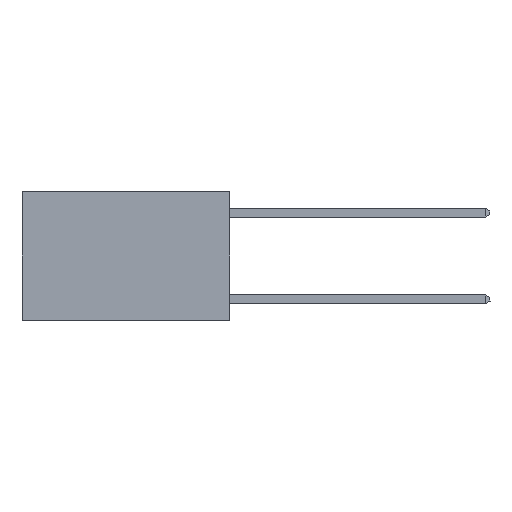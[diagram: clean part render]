
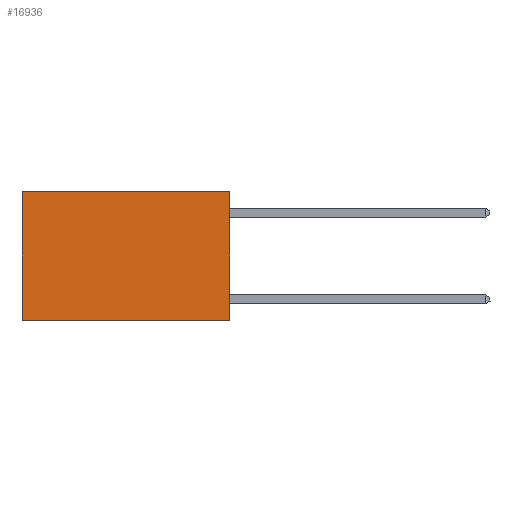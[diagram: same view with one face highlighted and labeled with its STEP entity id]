
A CAD part, left-side view. The second image highlights one B-rep face of the part: STEP entity #16936.
In plain terms, the highlighted planar face has unit normal (-1, 0, 0).
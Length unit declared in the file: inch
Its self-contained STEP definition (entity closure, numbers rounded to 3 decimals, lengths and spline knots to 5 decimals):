
#308 = ORIENTED_EDGE ( 'NONE', *, *, #13115, .T. ) ;
#621 = VERTEX_POINT ( 'NONE', #2435 ) ;
#2435 = CARTESIAN_POINT ( 'NONE',  ( 0.2625, 0., -0.37 ) ) ;
#2455 = VERTEX_POINT ( 'NONE', #16443 ) ;
#3854 = LINE ( 'NONE', #19638, #19950 ) ;
#4288 = DIRECTION ( 'NONE',  ( 0., 0., -1. ) ) ;
#4433 = LINE ( 'NONE', #13815, #7855 ) ;
#4659 = CARTESIAN_POINT ( 'NONE',  ( 0.2625, 0., 0. ) ) ;
#4822 = LINE ( 'NONE', #9016, #8762 ) ;
#6432 = PLANE ( 'NONE',  #19025 ) ;
#6442 = ORIENTED_EDGE ( 'NONE', *, *, #18600, .F. ) ;
#7121 = ORIENTED_EDGE ( 'NONE', *, *, #7258, .F. ) ;
#7258 = EDGE_CURVE ( 'NONE', #14819, #621, #4822, .T. ) ;
#7855 = VECTOR ( 'NONE', #15471, 39.37008 ) ;
#8762 = VECTOR ( 'NONE', #20571, 39.37008 ) ;
#9016 = CARTESIAN_POINT ( 'NONE',  ( 0.2625, 0., 0. ) ) ;
#9351 = CARTESIAN_POINT ( 'NONE',  ( 0.2625, 0.6, 0. ) ) ;
#9786 = DIRECTION ( 'NONE',  ( 1., 0., 0. ) ) ;
#10000 = CARTESIAN_POINT ( 'NONE',  ( 0.2625, 0.6, -0.37 ) ) ;
#11943 = LINE ( 'NONE', #9351, #15819 ) ;
#13093 = DIRECTION ( 'NONE',  ( 0., 1., 0. ) ) ;
#13115 = EDGE_CURVE ( 'NONE', #2455, #15050, #11943, .T. ) ;
#13815 = CARTESIAN_POINT ( 'NONE',  ( 0.2625, 0., 0. ) ) ;
#14245 = CARTESIAN_POINT ( 'NONE',  ( 0.2625, 0., 0. ) ) ;
#14819 = VERTEX_POINT ( 'NONE', #14245 ) ;
#15050 = VERTEX_POINT ( 'NONE', #10000 ) ;
#15471 = DIRECTION ( 'NONE',  ( 0., 1., 0. ) ) ;
#15819 = VECTOR ( 'NONE', #4288, 39.37008 ) ;
#16443 = CARTESIAN_POINT ( 'NONE',  ( 0.2625, 0.6, 0. ) ) ;
#16548 = EDGE_CURVE ( 'NONE', #14819, #2455, #4433, .T. ) ;
#16727 = EDGE_LOOP ( 'NONE', ( #308, #6442, #7121, #17987 ) ) ;
#16936 = ADVANCED_FACE ( 'NONE', ( #17171 ), #6432, .F. ) ;
#17171 = FACE_OUTER_BOUND ( 'NONE', #16727, .T. ) ;
#17987 = ORIENTED_EDGE ( 'NONE', *, *, #16548, .T. ) ;
#18600 = EDGE_CURVE ( 'NONE', #621, #15050, #3854, .T. ) ;
#19025 = AXIS2_PLACEMENT_3D ( 'NONE', #4659, #9786, #21299 ) ;
#19638 = CARTESIAN_POINT ( 'NONE',  ( 0.2625, 0., -0.37 ) ) ;
#19950 = VECTOR ( 'NONE', #13093, 39.37008 ) ;
#20571 = DIRECTION ( 'NONE',  ( 0., 0., -1. ) ) ;
#21299 = DIRECTION ( 'NONE',  ( 0., 0., -1. ) ) ;
